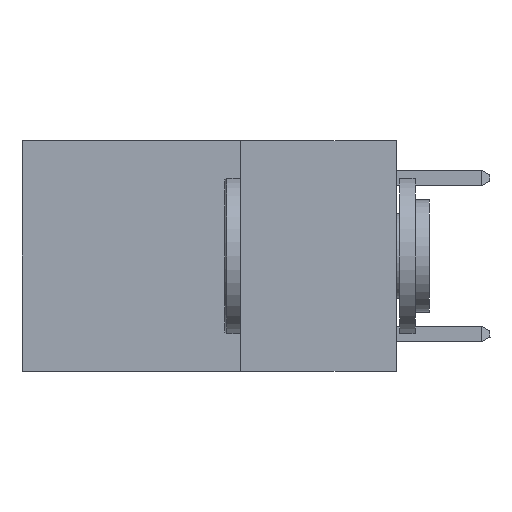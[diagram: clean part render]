
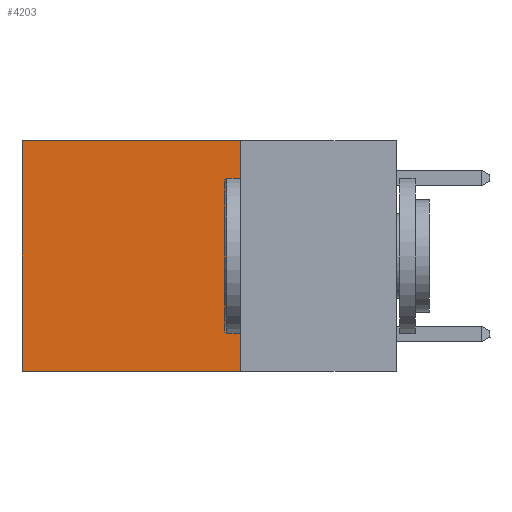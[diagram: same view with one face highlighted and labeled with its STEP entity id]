
A CAD part, left-side view. The second image highlights one B-rep face of the part: STEP entity #4203.
In plain terms, the highlighted planar face has unit normal (-1, 0, 0).
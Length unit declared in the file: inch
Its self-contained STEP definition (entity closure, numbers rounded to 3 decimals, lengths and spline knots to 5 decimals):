
#132 = VERTEX_POINT ( 'NONE', #4972 ) ;
#144 = ORIENTED_EDGE ( 'NONE', *, *, #12623, .T. ) ;
#177 = CARTESIAN_POINT ( 'NONE',  ( 0.2625, 0.6, 0. ) ) ;
#332 = EDGE_LOOP ( 'NONE', ( #144, #354, #715, #1830 ) ) ;
#354 = ORIENTED_EDGE ( 'NONE', *, *, #14217, .F. ) ;
#428 = CARTESIAN_POINT ( 'NONE',  ( 0.2625, 0.25, 0. ) ) ;
#454 = VERTEX_POINT ( 'NONE', #9307 ) ;
#558 = CARTESIAN_POINT ( 'NONE',  ( 0.2625, 0.25, 0. ) ) ;
#715 = ORIENTED_EDGE ( 'NONE', *, *, #2424, .F. ) ;
#1121 = DIRECTION ( 'NONE',  ( 0., 1., 0. ) ) ;
#1346 = DIRECTION ( 'NONE',  ( 0., 1., 0. ) ) ;
#1735 = EDGE_CURVE ( 'NONE', #454, #1824, #3917, .T. ) ;
#1824 = VERTEX_POINT ( 'NONE', #177 ) ;
#1830 = ORIENTED_EDGE ( 'NONE', *, *, #1735, .T. ) ;
#2424 = EDGE_CURVE ( 'NONE', #454, #11610, #13952, .T. ) ;
#2723 = CARTESIAN_POINT ( 'NONE',  ( 0.2625, 0.25, -0.37 ) ) ;
#2969 = DIRECTION ( 'NONE',  ( 0., 0., -1. ) ) ;
#3917 = LINE ( 'NONE', #10505, #9870 ) ;
#4203 = ADVANCED_FACE ( 'NONE', ( #14972 ), #10062, .F. ) ;
#4472 = DIRECTION ( 'NONE',  ( 0., 0., -1. ) ) ;
#4972 = CARTESIAN_POINT ( 'NONE',  ( 0.2625, 0.6, -0.37 ) ) ;
#5337 = DIRECTION ( 'NONE',  ( 1., 0., 0. ) ) ;
#6785 = AXIS2_PLACEMENT_3D ( 'NONE', #558, #5337, #13468 ) ;
#7292 = LINE ( 'NONE', #10611, #10070 ) ;
#8079 = CARTESIAN_POINT ( 'NONE',  ( 0.2625, 0.6, 0. ) ) ;
#8641 = LINE ( 'NONE', #8079, #13993 ) ;
#9307 = CARTESIAN_POINT ( 'NONE',  ( 0.2625, 0.25, 0. ) ) ;
#9870 = VECTOR ( 'NONE', #1346, 39.37008 ) ;
#10062 = PLANE ( 'NONE',  #6785 ) ;
#10070 = VECTOR ( 'NONE', #1121, 39.37008 ) ;
#10505 = CARTESIAN_POINT ( 'NONE',  ( 0.2625, 0.25, 0. ) ) ;
#10596 = VECTOR ( 'NONE', #2969, 39.37008 ) ;
#10611 = CARTESIAN_POINT ( 'NONE',  ( 0.2625, 0.25, -0.37 ) ) ;
#11610 = VERTEX_POINT ( 'NONE', #2723 ) ;
#12623 = EDGE_CURVE ( 'NONE', #1824, #132, #8641, .T. ) ;
#13468 = DIRECTION ( 'NONE',  ( 0., 0., -1. ) ) ;
#13952 = LINE ( 'NONE', #428, #10596 ) ;
#13993 = VECTOR ( 'NONE', #4472, 39.37008 ) ;
#14217 = EDGE_CURVE ( 'NONE', #11610, #132, #7292, .T. ) ;
#14972 = FACE_OUTER_BOUND ( 'NONE', #332, .T. ) ;
